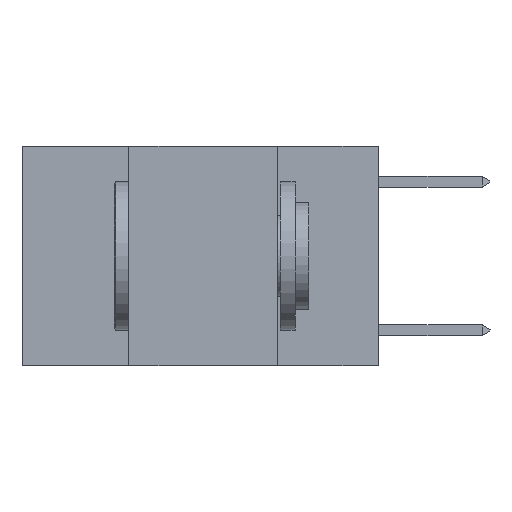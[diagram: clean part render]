
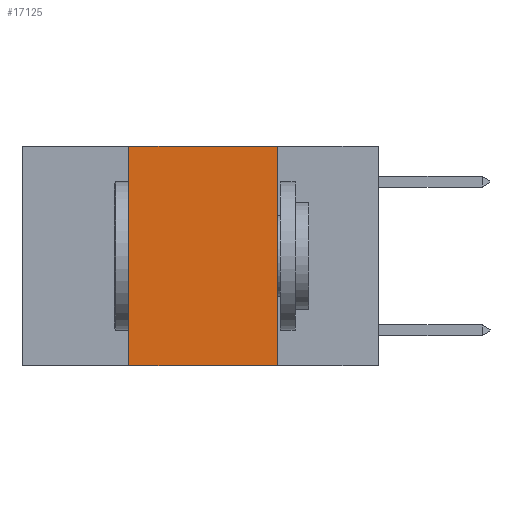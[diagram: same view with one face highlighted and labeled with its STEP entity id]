
A CAD part, left-side view. The second image highlights one B-rep face of the part: STEP entity #17125.
In plain terms, the highlighted planar face has unit normal (-1, 0, 0).
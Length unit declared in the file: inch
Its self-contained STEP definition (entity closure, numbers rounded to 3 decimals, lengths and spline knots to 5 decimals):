
#1171 = CARTESIAN_POINT ( 'NONE',  ( 0., 0.42, 0. ) ) ;
#2335 = CARTESIAN_POINT ( 'NONE',  ( 0., 0.17, 0. ) ) ;
#2396 = LINE ( 'NONE', #2335, #2621 ) ;
#2467 = ORIENTED_EDGE ( 'NONE', *, *, #17734, .F. ) ;
#2621 = VECTOR ( 'NONE', #15662, 39.37008 ) ;
#3414 = VERTEX_POINT ( 'NONE', #24871 ) ;
#4273 = EDGE_LOOP ( 'NONE', ( #2467, #26582, #26226, #4529 ) ) ;
#4410 = VECTOR ( 'NONE', #27023, 39.37008 ) ;
#4529 = ORIENTED_EDGE ( 'NONE', *, *, #9470, .T. ) ;
#4643 = PLANE ( 'NONE',  #16563 ) ;
#9164 = DIRECTION ( 'NONE',  ( 1., 0., 0. ) ) ;
#9470 = EDGE_CURVE ( 'NONE', #10261, #3414, #10273, .T. ) ;
#9521 = VECTOR ( 'NONE', #12494, 39.37008 ) ;
#10261 = VERTEX_POINT ( 'NONE', #22781 ) ;
#10273 = LINE ( 'NONE', #12589, #9521 ) ;
#11001 = FACE_OUTER_BOUND ( 'NONE', #4273, .T. ) ;
#11056 = LINE ( 'NONE', #23034, #4410 ) ;
#12494 = DIRECTION ( 'NONE',  ( 0., -1., 0. ) ) ;
#12589 = CARTESIAN_POINT ( 'NONE',  ( 0., 0.6, -0.37 ) ) ;
#14451 = VERTEX_POINT ( 'NONE', #22256 ) ;
#14904 = VECTOR ( 'NONE', #26877, 39.37008 ) ;
#15662 = DIRECTION ( 'NONE',  ( 0., 0., -1. ) ) ;
#16563 = AXIS2_PLACEMENT_3D ( 'NONE', #22217, #9164, #24351 ) ;
#17125 = ADVANCED_FACE ( 'NONE', ( #11001 ), #4643, .F. ) ;
#17734 = EDGE_CURVE ( 'NONE', #14451, #3414, #2396, .T. ) ;
#18869 = VERTEX_POINT ( 'NONE', #1171 ) ;
#20218 = EDGE_CURVE ( 'NONE', #18869, #14451, #22014, .T. ) ;
#21168 = EDGE_CURVE ( 'NONE', #10261, #18869, #11056, .T. ) ;
#22014 = LINE ( 'NONE', #24795, #14904 ) ;
#22217 = CARTESIAN_POINT ( 'NONE',  ( 0., 0.6, 0. ) ) ;
#22256 = CARTESIAN_POINT ( 'NONE',  ( 0., 0.17, 0. ) ) ;
#22781 = CARTESIAN_POINT ( 'NONE',  ( 0., 0.42, -0.37 ) ) ;
#23034 = CARTESIAN_POINT ( 'NONE',  ( 0., 0.42, 0. ) ) ;
#24351 = DIRECTION ( 'NONE',  ( 0., 0., -1. ) ) ;
#24795 = CARTESIAN_POINT ( 'NONE',  ( 0., 0.6, 0. ) ) ;
#24871 = CARTESIAN_POINT ( 'NONE',  ( 0., 0.17, -0.37 ) ) ;
#26226 = ORIENTED_EDGE ( 'NONE', *, *, #21168, .F. ) ;
#26582 = ORIENTED_EDGE ( 'NONE', *, *, #20218, .F. ) ;
#26877 = DIRECTION ( 'NONE',  ( 0., -1., 0. ) ) ;
#27023 = DIRECTION ( 'NONE',  ( 0., 0., 1. ) ) ;
